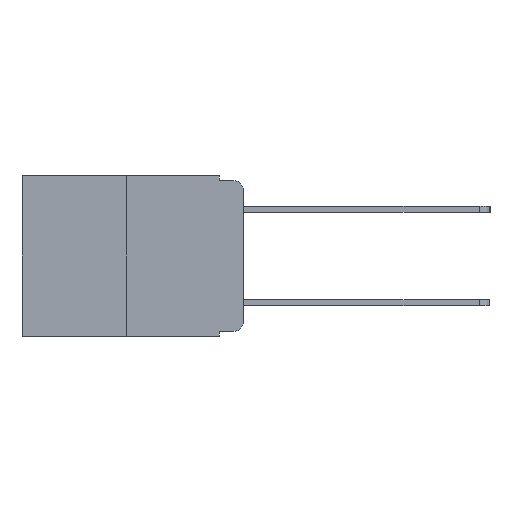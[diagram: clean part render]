
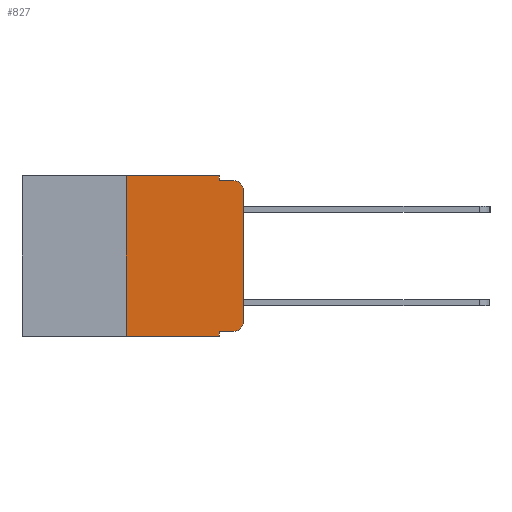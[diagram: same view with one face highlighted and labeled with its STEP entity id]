
A CAD part, left-side view. The second image highlights one B-rep face of the part: STEP entity #827.
In plain terms, the highlighted planar face has unit normal (-1, 0, 0).
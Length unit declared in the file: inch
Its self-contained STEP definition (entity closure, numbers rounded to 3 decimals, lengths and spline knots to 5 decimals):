
#190 = VECTOR ( 'NONE', #10336, 39.37008 ) ;
#570 = EDGE_CURVE ( 'NONE', #12593, #4136, #1153, .T. ) ;
#793 = VECTOR ( 'NONE', #11690, 39.37008 ) ;
#827 = ADVANCED_FACE ( 'NONE', ( #10979 ), #3846, .F. ) ;
#907 = CARTESIAN_POINT ( 'NONE',  ( 0., 0.25, 0. ) ) ;
#1019 = LINE ( 'NONE', #12658, #6625 ) ;
#1153 = LINE ( 'NONE', #8891, #8691 ) ;
#1186 = CARTESIAN_POINT ( 'NONE',  ( 0., 0.051, -0.333 ) ) ;
#1260 = CARTESIAN_POINT ( 'NONE',  ( 0., 0.02, -0.03 ) ) ;
#2104 = CARTESIAN_POINT ( 'NONE',  ( 0., 0.051, 0. ) ) ;
#2150 = CARTESIAN_POINT ( 'NONE',  ( 0., 0., -0.313 ) ) ;
#2167 = CIRCLE ( 'NONE', #11891, 0.02 ) ;
#2188 = DIRECTION ( 'NONE',  ( 0., 0., 1. ) ) ;
#2360 = CARTESIAN_POINT ( 'NONE',  ( 0., 0.051, -0.01 ) ) ;
#2510 = DIRECTION ( 'NONE',  ( 0., 0., -1. ) ) ;
#2666 = ORIENTED_EDGE ( 'NONE', *, *, #11674, .T. ) ;
#2901 = CARTESIAN_POINT ( 'NONE',  ( 0., 0.25, -0.343 ) ) ;
#2935 = CARTESIAN_POINT ( 'NONE',  ( 0., 0.051, -0.333 ) ) ;
#3399 = VECTOR ( 'NONE', #10547, 39.37008 ) ;
#3446 = LINE ( 'NONE', #2104, #190 ) ;
#3495 = CARTESIAN_POINT ( 'NONE',  ( 0., 0., 0. ) ) ;
#3846 = PLANE ( 'NONE',  #12038 ) ;
#3975 = LINE ( 'NONE', #4691, #793 ) ;
#4085 = ORIENTED_EDGE ( 'NONE', *, *, #5786, .T. ) ;
#4129 = CARTESIAN_POINT ( 'NONE',  ( 0., 0., -0.03 ) ) ;
#4136 = VERTEX_POINT ( 'NONE', #9298 ) ;
#4173 = VERTEX_POINT ( 'NONE', #10305 ) ;
#4691 = CARTESIAN_POINT ( 'NONE',  ( 0., 0.473, 0. ) ) ;
#5156 = DIRECTION ( 'NONE',  ( 0., -1., 0. ) ) ;
#5786 = EDGE_CURVE ( 'NONE', #9582, #9170, #7113, .T. ) ;
#6150 = VECTOR ( 'NONE', #7856, 39.37008 ) ;
#6271 = LINE ( 'NONE', #3495, #3399 ) ;
#6552 = CARTESIAN_POINT ( 'NONE',  ( 0., 0.02, -0.313 ) ) ;
#6625 = VECTOR ( 'NONE', #7746, 39.37008 ) ;
#6888 = CARTESIAN_POINT ( 'NONE',  ( 0., 0.051, -0.01 ) ) ;
#6925 = VECTOR ( 'NONE', #2188, 39.37008 ) ;
#6950 = VECTOR ( 'NONE', #5156, 39.37008 ) ;
#7105 = EDGE_CURVE ( 'NONE', #9346, #9582, #12431, .T. ) ;
#7113 = CIRCLE ( 'NONE', #7115, 0.02 ) ;
#7115 = AXIS2_PLACEMENT_3D ( 'NONE', #6552, #13350, #7522 ) ;
#7522 = DIRECTION ( 'NONE',  ( 0., 0., -1. ) ) ;
#7746 = DIRECTION ( 'NONE',  ( 0., 0., -1. ) ) ;
#7748 = EDGE_CURVE ( 'NONE', #9346, #4136, #1019, .T. ) ;
#7856 = DIRECTION ( 'NONE',  ( 0., -1., 0. ) ) ;
#7940 = CARTESIAN_POINT ( 'NONE',  ( 0., 0.25, 0. ) ) ;
#8101 = VERTEX_POINT ( 'NONE', #4129 ) ;
#8282 = VERTEX_POINT ( 'NONE', #8343 ) ;
#8343 = CARTESIAN_POINT ( 'NONE',  ( 0., 0.051, 0. ) ) ;
#8409 = EDGE_CURVE ( 'NONE', #12593, #13333, #9205, .T. ) ;
#8691 = VECTOR ( 'NONE', #10314, 39.37008 ) ;
#8720 = LINE ( 'NONE', #6888, #6150 ) ;
#8736 = DIRECTION ( 'NONE',  ( -1., 0., 0. ) ) ;
#8812 = CARTESIAN_POINT ( 'NONE',  ( 0., 0.473, 0. ) ) ;
#8823 = ORIENTED_EDGE ( 'NONE', *, *, #10358, .F. ) ;
#8891 = CARTESIAN_POINT ( 'NONE',  ( 0., 0.473, -0.343 ) ) ;
#8991 = ORIENTED_EDGE ( 'NONE', *, *, #10282, .F. ) ;
#9006 = ORIENTED_EDGE ( 'NONE', *, *, #7748, .F. ) ;
#9073 = EDGE_CURVE ( 'NONE', #8282, #10924, #3446, .T. ) ;
#9170 = VERTEX_POINT ( 'NONE', #2150 ) ;
#9205 = LINE ( 'NONE', #907, #6925 ) ;
#9298 = CARTESIAN_POINT ( 'NONE',  ( 0., 0.051, -0.343 ) ) ;
#9346 = VERTEX_POINT ( 'NONE', #1186 ) ;
#9582 = VERTEX_POINT ( 'NONE', #10847 ) ;
#10192 = ORIENTED_EDGE ( 'NONE', *, *, #8409, .F. ) ;
#10282 = EDGE_CURVE ( 'NONE', #13333, #8282, #3975, .T. ) ;
#10305 = CARTESIAN_POINT ( 'NONE',  ( 0., 0.02, -0.01 ) ) ;
#10314 = DIRECTION ( 'NONE',  ( 0., -1., 0. ) ) ;
#10336 = DIRECTION ( 'NONE',  ( 0., 0., -1. ) ) ;
#10358 = EDGE_CURVE ( 'NONE', #10924, #4173, #8720, .T. ) ;
#10547 = DIRECTION ( 'NONE',  ( 0., 0., 1. ) ) ;
#10797 = ORIENTED_EDGE ( 'NONE', *, *, #11023, .T. ) ;
#10847 = CARTESIAN_POINT ( 'NONE',  ( 0., 0.02, -0.333 ) ) ;
#10924 = VERTEX_POINT ( 'NONE', #2360 ) ;
#10979 = FACE_OUTER_BOUND ( 'NONE', #11048, .T. ) ;
#11023 = EDGE_CURVE ( 'NONE', #8101, #4173, #2167, .T. ) ;
#11048 = EDGE_LOOP ( 'NONE', ( #2666, #10797, #8823, #11720, #8991, #10192, #12650, #9006, #11119, #4085 ) ) ;
#11119 = ORIENTED_EDGE ( 'NONE', *, *, #7105, .T. ) ;
#11674 = EDGE_CURVE ( 'NONE', #9170, #8101, #6271, .T. ) ;
#11690 = DIRECTION ( 'NONE',  ( 0., -1., 0. ) ) ;
#11720 = ORIENTED_EDGE ( 'NONE', *, *, #9073, .F. ) ;
#11891 = AXIS2_PLACEMENT_3D ( 'NONE', #1260, #8736, #2510 ) ;
#12038 = AXIS2_PLACEMENT_3D ( 'NONE', #8812, #13101, #12121 ) ;
#12121 = DIRECTION ( 'NONE',  ( 0., 0., -1. ) ) ;
#12431 = LINE ( 'NONE', #2935, #6950 ) ;
#12593 = VERTEX_POINT ( 'NONE', #2901 ) ;
#12650 = ORIENTED_EDGE ( 'NONE', *, *, #570, .T. ) ;
#12658 = CARTESIAN_POINT ( 'NONE',  ( 0., 0.051, 0. ) ) ;
#13101 = DIRECTION ( 'NONE',  ( 1., 0., 0. ) ) ;
#13333 = VERTEX_POINT ( 'NONE', #7940 ) ;
#13350 = DIRECTION ( 'NONE',  ( -1., 0., 0. ) ) ;
